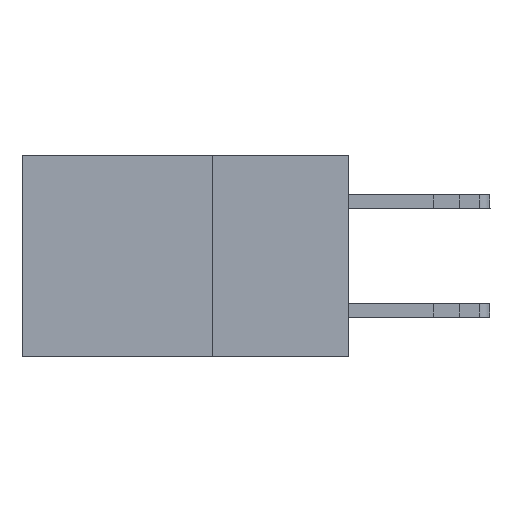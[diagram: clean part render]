
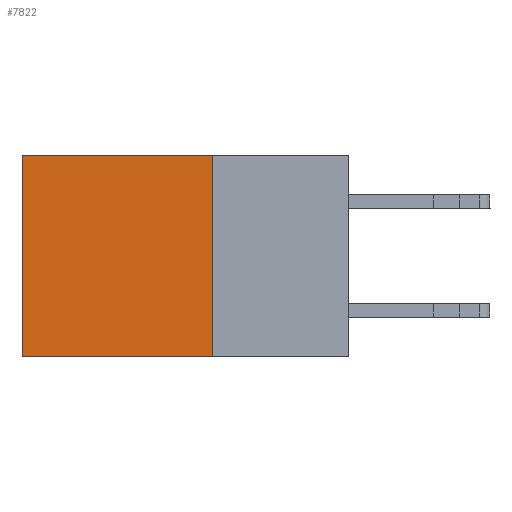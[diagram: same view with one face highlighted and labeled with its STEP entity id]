
A CAD part, left-side view. The second image highlights one B-rep face of the part: STEP entity #7822.
In plain terms, the highlighted planar face has unit normal (-1, 0, 0).
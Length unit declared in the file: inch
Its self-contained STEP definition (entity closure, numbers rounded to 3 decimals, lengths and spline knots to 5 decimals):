
#28 = VECTOR ( 'NONE', #9150, 39.37008 ) ;
#741 = CARTESIAN_POINT ( 'NONE',  ( 0.298, 0.25, 0. ) ) ;
#744 = DIRECTION ( 'NONE',  ( 0., 1., 0. ) ) ;
#2666 = CARTESIAN_POINT ( 'NONE',  ( 0.298, 0.25, 0. ) ) ;
#2712 = DIRECTION ( 'NONE',  ( 0., 0., -1. ) ) ;
#2737 = DIRECTION ( 'NONE',  ( 0., 1., 0. ) ) ;
#3216 = CARTESIAN_POINT ( 'NONE',  ( 0.298, 0.25, 0. ) ) ;
#3438 = EDGE_LOOP ( 'NONE', ( #12265, #11625, #6234, #9590 ) ) ;
#4695 = EDGE_CURVE ( 'NONE', #5706, #12110, #10333, .T. ) ;
#4772 = VERTEX_POINT ( 'NONE', #5481 ) ;
#4847 = CARTESIAN_POINT ( 'NONE',  ( 0.298, 0.25, 0. ) ) ;
#4963 = EDGE_CURVE ( 'NONE', #4772, #7382, #6830, .T. ) ;
#5206 = VECTOR ( 'NONE', #744, 39.37008 ) ;
#5481 = CARTESIAN_POINT ( 'NONE',  ( 0.298, 0.6, 0. ) ) ;
#5531 = VECTOR ( 'NONE', #2712, 39.37008 ) ;
#5686 = CARTESIAN_POINT ( 'NONE',  ( 0.298, 0.25, -0.37 ) ) ;
#5706 = VERTEX_POINT ( 'NONE', #741 ) ;
#5772 = DIRECTION ( 'NONE',  ( 1., 0., 0. ) ) ;
#6234 = ORIENTED_EDGE ( 'NONE', *, *, #4695, .F. ) ;
#6784 = DIRECTION ( 'NONE',  ( 0., 0., -1. ) ) ;
#6830 = LINE ( 'NONE', #8964, #5531 ) ;
#6852 = LINE ( 'NONE', #9835, #5206 ) ;
#7382 = VERTEX_POINT ( 'NONE', #9730 ) ;
#7727 = LINE ( 'NONE', #4847, #8897 ) ;
#7822 = ADVANCED_FACE ( 'NONE', ( #12889 ), #11755, .F. ) ;
#8897 = VECTOR ( 'NONE', #2737, 39.37008 ) ;
#8964 = CARTESIAN_POINT ( 'NONE',  ( 0.298, 0.6, 0. ) ) ;
#9150 = DIRECTION ( 'NONE',  ( 0., 0., -1. ) ) ;
#9152 = EDGE_CURVE ( 'NONE', #12110, #7382, #6852, .T. ) ;
#9590 = ORIENTED_EDGE ( 'NONE', *, *, #10429, .T. ) ;
#9730 = CARTESIAN_POINT ( 'NONE',  ( 0.298, 0.6, -0.37 ) ) ;
#9835 = CARTESIAN_POINT ( 'NONE',  ( 0.298, 0.25, -0.37 ) ) ;
#10333 = LINE ( 'NONE', #3216, #28 ) ;
#10429 = EDGE_CURVE ( 'NONE', #5706, #4772, #7727, .T. ) ;
#11625 = ORIENTED_EDGE ( 'NONE', *, *, #9152, .F. ) ;
#11755 = PLANE ( 'NONE',  #12198 ) ;
#12110 = VERTEX_POINT ( 'NONE', #5686 ) ;
#12198 = AXIS2_PLACEMENT_3D ( 'NONE', #2666, #5772, #6784 ) ;
#12265 = ORIENTED_EDGE ( 'NONE', *, *, #4963, .T. ) ;
#12889 = FACE_OUTER_BOUND ( 'NONE', #3438, .T. ) ;
